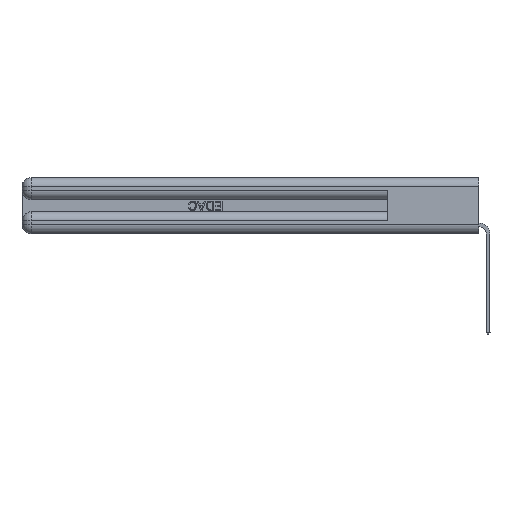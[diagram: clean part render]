
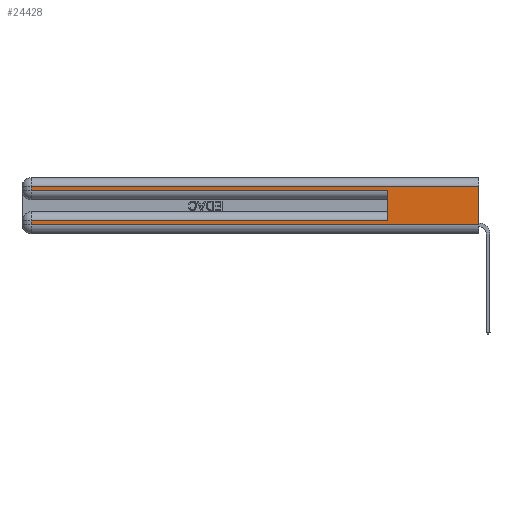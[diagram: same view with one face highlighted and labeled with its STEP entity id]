
A CAD part, left-side view. The second image highlights one B-rep face of the part: STEP entity #24428.
In plain terms, the highlighted planar face has unit normal (-1, 0, 0).
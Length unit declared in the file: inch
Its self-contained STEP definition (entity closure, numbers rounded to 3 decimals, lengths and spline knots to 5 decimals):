
#705 = VECTOR ( 'NONE', #27126, 39.37008 ) ;
#727 = VERTEX_POINT ( 'NONE', #3719 ) ;
#944 = EDGE_CURVE ( 'NONE', #16630, #6625, #18588, .T. ) ;
#1120 = DIRECTION ( 'NONE',  ( 0., 0., -1. ) ) ;
#2020 = VECTOR ( 'NONE', #8804, 39.37008 ) ;
#2189 = EDGE_LOOP ( 'NONE', ( #5076, #3760, #8766, #25107, #5614, #15619, #9094, #27556 ) ) ;
#2594 = LINE ( 'NONE', #11318, #15170 ) ;
#2706 = VECTOR ( 'NONE', #12188, 39.37008 ) ;
#2814 = DIRECTION ( 'NONE',  ( 0., 0., -1. ) ) ;
#3719 = CARTESIAN_POINT ( 'NONE',  ( 0., 0.6, 0.085 ) ) ;
#3760 = ORIENTED_EDGE ( 'NONE', *, *, #13977, .T. ) ;
#3962 = EDGE_CURVE ( 'NONE', #26716, #4142, #13534, .T. ) ;
#4142 = VERTEX_POINT ( 'NONE', #19287 ) ;
#4729 = CARTESIAN_POINT ( 'NONE',  ( 0., 2.94, 0.31 ) ) ;
#5061 = CARTESIAN_POINT ( 'NONE',  ( 0., 2.94, 0.37 ) ) ;
#5076 = ORIENTED_EDGE ( 'NONE', *, *, #20872, .F. ) ;
#5123 = EDGE_CURVE ( 'NONE', #727, #26716, #16524, .T. ) ;
#5614 = ORIENTED_EDGE ( 'NONE', *, *, #25372, .F. ) ;
#6028 = DIRECTION ( 'NONE',  ( 0., 1., 0. ) ) ;
#6625 = VERTEX_POINT ( 'NONE', #21372 ) ;
#8766 = ORIENTED_EDGE ( 'NONE', *, *, #26106, .T. ) ;
#8804 = DIRECTION ( 'NONE',  ( 0., 0., 1. ) ) ;
#9094 = ORIENTED_EDGE ( 'NONE', *, *, #3962, .T. ) ;
#9356 = VECTOR ( 'NONE', #6028, 39.37008 ) ;
#9616 = CARTESIAN_POINT ( 'NONE',  ( 0., 0., 0.085 ) ) ;
#11318 = CARTESIAN_POINT ( 'NONE',  ( 0., 0., 0.06 ) ) ;
#12132 = FACE_OUTER_BOUND ( 'NONE', #2189, .T. ) ;
#12141 = VECTOR ( 'NONE', #13200, 39.37008 ) ;
#12188 = DIRECTION ( 'NONE',  ( 0., 1., 0. ) ) ;
#13200 = DIRECTION ( 'NONE',  ( 0., 0., -1. ) ) ;
#13534 = LINE ( 'NONE', #13682, #26505 ) ;
#13682 = CARTESIAN_POINT ( 'NONE',  ( 0., 2.94, 0.37 ) ) ;
#13977 = EDGE_CURVE ( 'NONE', #19030, #19791, #21094, .T. ) ;
#14234 = VERTEX_POINT ( 'NONE', #21157 ) ;
#14290 = LINE ( 'NONE', #27838, #14335 ) ;
#14301 = PLANE ( 'NONE',  #18521 ) ;
#14335 = VECTOR ( 'NONE', #23073, 39.37008 ) ;
#15170 = VECTOR ( 'NONE', #21841, 39.37008 ) ;
#15619 = ORIENTED_EDGE ( 'NONE', *, *, #5123, .T. ) ;
#16496 = CARTESIAN_POINT ( 'NONE',  ( 0., 2.94, 0.285 ) ) ;
#16524 = LINE ( 'NONE', #9616, #2706 ) ;
#16630 = VERTEX_POINT ( 'NONE', #16496 ) ;
#17711 = CARTESIAN_POINT ( 'NONE',  ( 0., 0.6, 0.145 ) ) ;
#18170 = CARTESIAN_POINT ( 'NONE',  ( 0., 0., 0.31 ) ) ;
#18324 = CARTESIAN_POINT ( 'NONE',  ( 0., 0., 0.285 ) ) ;
#18521 = AXIS2_PLACEMENT_3D ( 'NONE', #20758, #27572, #1120 ) ;
#18588 = LINE ( 'NONE', #18324, #705 ) ;
#18778 = EDGE_CURVE ( 'NONE', #4142, #14234, #2594, .T. ) ;
#19030 = VERTEX_POINT ( 'NONE', #18170 ) ;
#19287 = CARTESIAN_POINT ( 'NONE',  ( 0., 2.94, 0.06 ) ) ;
#19791 = VERTEX_POINT ( 'NONE', #4729 ) ;
#19865 = LINE ( 'NONE', #17711, #2020 ) ;
#20758 = CARTESIAN_POINT ( 'NONE',  ( 0., 0., 0.37 ) ) ;
#20872 = EDGE_CURVE ( 'NONE', #19030, #14234, #14290, .T. ) ;
#21094 = LINE ( 'NONE', #25858, #9356 ) ;
#21157 = CARTESIAN_POINT ( 'NONE',  ( 0., 0., 0.06 ) ) ;
#21372 = CARTESIAN_POINT ( 'NONE',  ( 0., 0.6, 0.285 ) ) ;
#21841 = DIRECTION ( 'NONE',  ( 0., -1., 0. ) ) ;
#23073 = DIRECTION ( 'NONE',  ( 0., 0., -1. ) ) ;
#24428 = ADVANCED_FACE ( 'NONE', ( #12132 ), #14301, .F. ) ;
#24757 = LINE ( 'NONE', #5061, #12141 ) ;
#25107 = ORIENTED_EDGE ( 'NONE', *, *, #944, .T. ) ;
#25372 = EDGE_CURVE ( 'NONE', #727, #6625, #19865, .T. ) ;
#25858 = CARTESIAN_POINT ( 'NONE',  ( 0., 0., 0.31 ) ) ;
#26106 = EDGE_CURVE ( 'NONE', #19791, #16630, #24757, .T. ) ;
#26505 = VECTOR ( 'NONE', #2814, 39.37008 ) ;
#26716 = VERTEX_POINT ( 'NONE', #26964 ) ;
#26964 = CARTESIAN_POINT ( 'NONE',  ( 0., 2.94, 0.085 ) ) ;
#27126 = DIRECTION ( 'NONE',  ( 0., -1., 0. ) ) ;
#27556 = ORIENTED_EDGE ( 'NONE', *, *, #18778, .T. ) ;
#27572 = DIRECTION ( 'NONE',  ( 1., 0., 0. ) ) ;
#27838 = CARTESIAN_POINT ( 'NONE',  ( 0., 0., 0.37 ) ) ;
